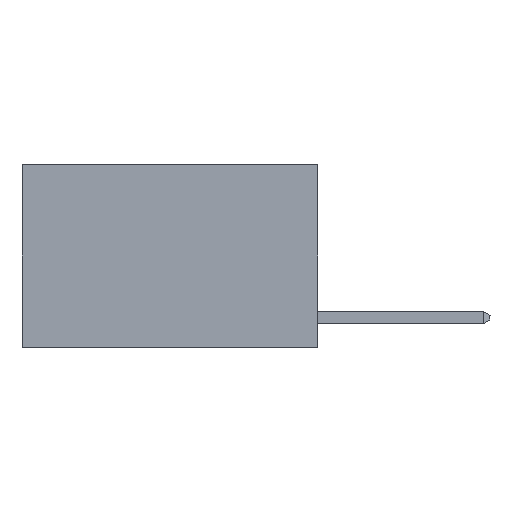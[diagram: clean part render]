
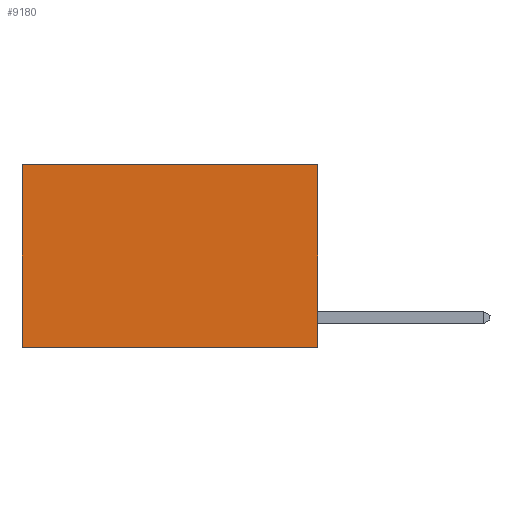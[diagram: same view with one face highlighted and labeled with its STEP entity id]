
A CAD part, left-side view. The second image highlights one B-rep face of the part: STEP entity #9180.
In plain terms, the highlighted planar face has unit normal (-1, 0, 0).
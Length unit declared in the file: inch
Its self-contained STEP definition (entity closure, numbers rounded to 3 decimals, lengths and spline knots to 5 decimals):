
#129 = CARTESIAN_POINT ( 'NONE',  ( 0.2625, 0., 0. ) ) ;
#557 = EDGE_CURVE ( 'NONE', #7851, #8546, #8473, .T. ) ;
#1513 = EDGE_LOOP ( 'NONE', ( #3914, #6303, #3864, #11691 ) ) ;
#1586 = VECTOR ( 'NONE', #10752, 39.37008 ) ;
#2042 = DIRECTION ( 'NONE',  ( 0., 0., -1. ) ) ;
#2207 = CARTESIAN_POINT ( 'NONE',  ( 0.2625, 0., 0. ) ) ;
#2333 = CARTESIAN_POINT ( 'NONE',  ( 0.2625, 0., 0. ) ) ;
#2782 = CARTESIAN_POINT ( 'NONE',  ( 0.2625, 0.6, -0.37 ) ) ;
#2990 = EDGE_CURVE ( 'NONE', #11611, #8546, #8073, .T. ) ;
#3462 = VECTOR ( 'NONE', #4864, 39.37008 ) ;
#3864 = ORIENTED_EDGE ( 'NONE', *, *, #7245, .F. ) ;
#3914 = ORIENTED_EDGE ( 'NONE', *, *, #557, .T. ) ;
#3941 = FACE_OUTER_BOUND ( 'NONE', #1513, .T. ) ;
#4205 = CARTESIAN_POINT ( 'NONE',  ( 0.2625, 0., 0. ) ) ;
#4223 = DIRECTION ( 'NONE',  ( 1., 0., 0. ) ) ;
#4864 = DIRECTION ( 'NONE',  ( 0., 0., -1. ) ) ;
#5325 = PLANE ( 'NONE',  #6486 ) ;
#6303 = ORIENTED_EDGE ( 'NONE', *, *, #2990, .F. ) ;
#6486 = AXIS2_PLACEMENT_3D ( 'NONE', #2333, #4223, #9946 ) ;
#6805 = CARTESIAN_POINT ( 'NONE',  ( 0.2625, 0., -0.37 ) ) ;
#7245 = EDGE_CURVE ( 'NONE', #11336, #11611, #10866, .T. ) ;
#7750 = DIRECTION ( 'NONE',  ( 0., 1., 0. ) ) ;
#7851 = VERTEX_POINT ( 'NONE', #9741 ) ;
#7927 = LINE ( 'NONE', #4205, #1586 ) ;
#8073 = LINE ( 'NONE', #6805, #9075 ) ;
#8473 = LINE ( 'NONE', #11936, #3462 ) ;
#8546 = VERTEX_POINT ( 'NONE', #2782 ) ;
#9075 = VECTOR ( 'NONE', #7750, 39.37008 ) ;
#9180 = ADVANCED_FACE ( 'NONE', ( #3941 ), #5325, .F. ) ;
#9741 = CARTESIAN_POINT ( 'NONE',  ( 0.2625, 0.6, 0. ) ) ;
#9946 = DIRECTION ( 'NONE',  ( 0., 0., -1. ) ) ;
#10306 = VECTOR ( 'NONE', #2042, 39.37008 ) ;
#10752 = DIRECTION ( 'NONE',  ( 0., 1., 0. ) ) ;
#10866 = LINE ( 'NONE', #129, #10306 ) ;
#11165 = CARTESIAN_POINT ( 'NONE',  ( 0.2625, 0., -0.37 ) ) ;
#11336 = VERTEX_POINT ( 'NONE', #2207 ) ;
#11611 = VERTEX_POINT ( 'NONE', #11165 ) ;
#11691 = ORIENTED_EDGE ( 'NONE', *, *, #12034, .T. ) ;
#11936 = CARTESIAN_POINT ( 'NONE',  ( 0.2625, 0.6, 0. ) ) ;
#12034 = EDGE_CURVE ( 'NONE', #11336, #7851, #7927, .T. ) ;
